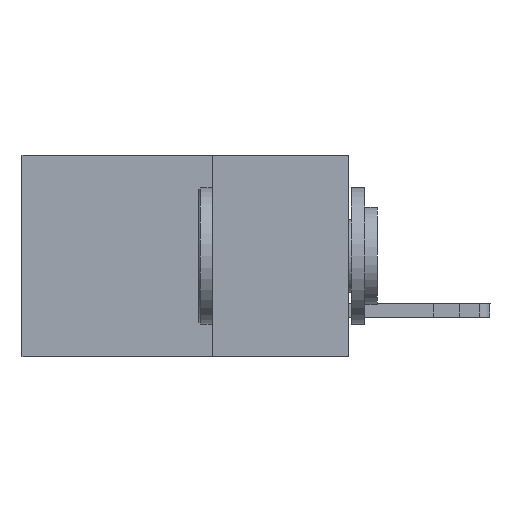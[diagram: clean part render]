
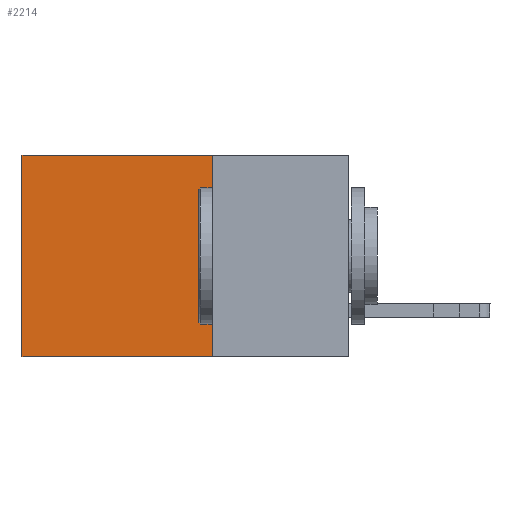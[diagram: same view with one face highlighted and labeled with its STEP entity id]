
A CAD part, left-side view. The second image highlights one B-rep face of the part: STEP entity #2214.
In plain terms, the highlighted planar face has unit normal (-1, 0, 0).
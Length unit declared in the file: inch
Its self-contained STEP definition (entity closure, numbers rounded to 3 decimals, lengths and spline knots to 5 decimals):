
#79 = VECTOR ( 'NONE', #3119, 39.37008 ) ;
#152 = VERTEX_POINT ( 'NONE', #12976 ) ;
#871 = VECTOR ( 'NONE', #7960, 39.37008 ) ;
#1703 = DIRECTION ( 'NONE',  ( 1., 0., 0. ) ) ;
#2154 = CARTESIAN_POINT ( 'NONE',  ( 0.298, 0.25, -0.37 ) ) ;
#2214 = ADVANCED_FACE ( 'NONE', ( #17011 ), #10717, .F. ) ;
#2800 = EDGE_CURVE ( 'NONE', #152, #17741, #13012, .T. ) ;
#3119 = DIRECTION ( 'NONE',  ( 0., 0., -1. ) ) ;
#3718 = CARTESIAN_POINT ( 'NONE',  ( 0.298, 0.25, 0. ) ) ;
#4537 = EDGE_CURVE ( 'NONE', #17741, #14934, #16709, .T. ) ;
#4550 = CARTESIAN_POINT ( 'NONE',  ( 0.298, 0.25, 0. ) ) ;
#4573 = VECTOR ( 'NONE', #9648, 39.37008 ) ;
#5182 = LINE ( 'NONE', #12150, #6488 ) ;
#5518 = EDGE_LOOP ( 'NONE', ( #12317, #9948, #13756, #16499 ) ) ;
#5711 = EDGE_CURVE ( 'NONE', #10926, #14934, #15306, .T. ) ;
#6488 = VECTOR ( 'NONE', #8362, 39.37008 ) ;
#7378 = CARTESIAN_POINT ( 'NONE',  ( 0.298, 0.6, 0. ) ) ;
#7960 = DIRECTION ( 'NONE',  ( 0., 0., -1. ) ) ;
#8288 = DIRECTION ( 'NONE',  ( 0., 0., -1. ) ) ;
#8362 = DIRECTION ( 'NONE',  ( 0., 1., 0. ) ) ;
#9648 = DIRECTION ( 'NONE',  ( 0., 1., 0. ) ) ;
#9948 = ORIENTED_EDGE ( 'NONE', *, *, #4537, .F. ) ;
#10322 = CARTESIAN_POINT ( 'NONE',  ( 0.298, 0.6, -0.37 ) ) ;
#10717 = PLANE ( 'NONE',  #18195 ) ;
#10926 = VERTEX_POINT ( 'NONE', #16946 ) ;
#12150 = CARTESIAN_POINT ( 'NONE',  ( 0.298, 0.25, 0. ) ) ;
#12317 = ORIENTED_EDGE ( 'NONE', *, *, #5711, .T. ) ;
#12524 = EDGE_CURVE ( 'NONE', #152, #10926, #5182, .T. ) ;
#12976 = CARTESIAN_POINT ( 'NONE',  ( 0.298, 0.25, 0. ) ) ;
#13012 = LINE ( 'NONE', #4550, #871 ) ;
#13756 = ORIENTED_EDGE ( 'NONE', *, *, #2800, .F. ) ;
#14934 = VERTEX_POINT ( 'NONE', #10322 ) ;
#15306 = LINE ( 'NONE', #7378, #79 ) ;
#16499 = ORIENTED_EDGE ( 'NONE', *, *, #12524, .T. ) ;
#16709 = LINE ( 'NONE', #2154, #4573 ) ;
#16804 = CARTESIAN_POINT ( 'NONE',  ( 0.298, 0.25, -0.37 ) ) ;
#16946 = CARTESIAN_POINT ( 'NONE',  ( 0.298, 0.6, 0. ) ) ;
#17011 = FACE_OUTER_BOUND ( 'NONE', #5518, .T. ) ;
#17741 = VERTEX_POINT ( 'NONE', #16804 ) ;
#18195 = AXIS2_PLACEMENT_3D ( 'NONE', #3718, #1703, #8288 ) ;
